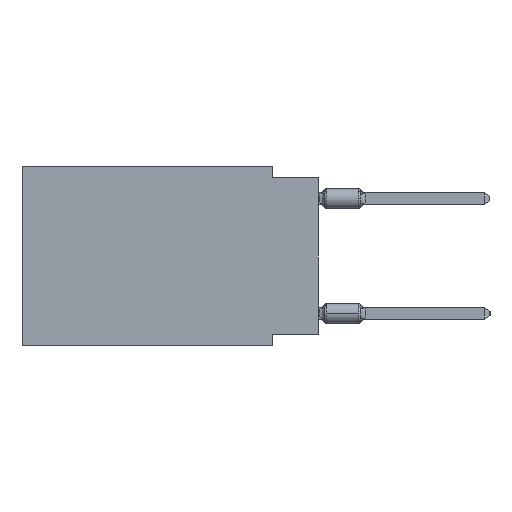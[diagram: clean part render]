
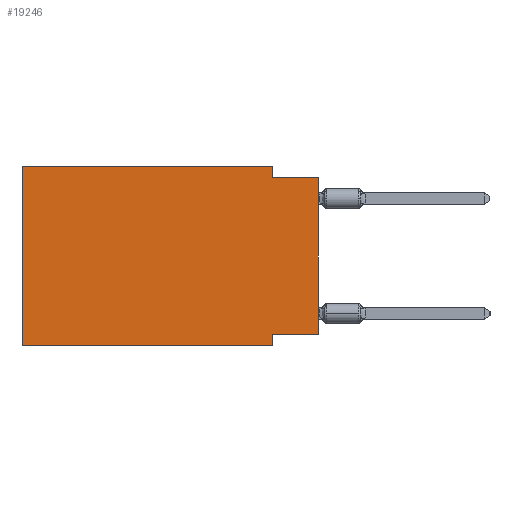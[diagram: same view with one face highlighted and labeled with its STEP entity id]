
A CAD part, left-side view. The second image highlights one B-rep face of the part: STEP entity #19246.
In plain terms, the highlighted planar face has unit normal (-1, 0, 0).
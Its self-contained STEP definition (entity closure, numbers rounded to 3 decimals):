
#781 = DIRECTION ( 'NONE',  ( 0., 1., 0. ) ) ;
#1164 = LINE ( 'NONE', #32238, #18415 ) ;
#2078 = VERTEX_POINT ( 'NONE', #16700 ) ;
#3327 = VERTEX_POINT ( 'NONE', #29608 ) ;
#3727 = CARTESIAN_POINT ( 'NONE',  ( 0., 16.383, -9.906 ) ) ;
#4197 = CARTESIAN_POINT ( 'NONE',  ( 0., 16.383, 0. ) ) ;
#5447 = CARTESIAN_POINT ( 'NONE',  ( 0., 2.54, -9.906 ) ) ;
#6340 = DIRECTION ( 'NONE',  ( 0., -1., 0. ) ) ;
#6601 = EDGE_CURVE ( 'NONE', #8725, #21561, #20114, .T. ) ;
#6744 = CARTESIAN_POINT ( 'NONE',  ( 0., 0., -9.271 ) ) ;
#7801 = CARTESIAN_POINT ( 'NONE',  ( 0., 2.54, 0. ) ) ;
#8725 = VERTEX_POINT ( 'NONE', #10551 ) ;
#9863 = EDGE_CURVE ( 'NONE', #2078, #21561, #28141, .T. ) ;
#9969 = DIRECTION ( 'NONE',  ( 0., 0., 1. ) ) ;
#9999 = EDGE_CURVE ( 'NONE', #13190, #2078, #26656, .T. ) ;
#10115 = VERTEX_POINT ( 'NONE', #18653 ) ;
#10551 = CARTESIAN_POINT ( 'NONE',  ( 0., 16.383, -9.906 ) ) ;
#11182 = VECTOR ( 'NONE', #6340, 1000. ) ;
#12348 = DIRECTION ( 'NONE',  ( 0., 0., 1. ) ) ;
#12403 = PLANE ( 'NONE',  #26948 ) ;
#13190 = VERTEX_POINT ( 'NONE', #34183 ) ;
#13383 = DIRECTION ( 'NONE',  ( 0., 0., -1. ) ) ;
#14023 = CARTESIAN_POINT ( 'NONE',  ( 0., 2.54, -9.906 ) ) ;
#15368 = CARTESIAN_POINT ( 'NONE',  ( 0., 0., -0.635 ) ) ;
#15559 = DIRECTION ( 'NONE',  ( 1., 0., 0. ) ) ;
#15912 = CARTESIAN_POINT ( 'NONE',  ( 0., 0., -0.635 ) ) ;
#16056 = EDGE_CURVE ( 'NONE', #10115, #3327, #20407, .T. ) ;
#16066 = DIRECTION ( 'NONE',  ( 0., -1., 0. ) ) ;
#16265 = DIRECTION ( 'NONE',  ( 0., -1., 0. ) ) ;
#16700 = CARTESIAN_POINT ( 'NONE',  ( 0., 2.54, -9.271 ) ) ;
#16948 = CARTESIAN_POINT ( 'NONE',  ( 0., 2.54, -0.635 ) ) ;
#18415 = VECTOR ( 'NONE', #12348, 1000. ) ;
#18653 = CARTESIAN_POINT ( 'NONE',  ( 0., 16.383, 0. ) ) ;
#19138 = EDGE_CURVE ( 'NONE', #8725, #10115, #35087, .T. ) ;
#19246 = ADVANCED_FACE ( 'NONE', ( #26521 ), #12403, .F. ) ;
#19527 = LINE ( 'NONE', #7801, #29988 ) ;
#20114 = LINE ( 'NONE', #3727, #11182 ) ;
#20407 = LINE ( 'NONE', #29647, #36608 ) ;
#21187 = ORIENTED_EDGE ( 'NONE', *, *, #16056, .F. ) ;
#21561 = VERTEX_POINT ( 'NONE', #5447 ) ;
#22024 = LINE ( 'NONE', #15912, #30311 ) ;
#22177 = VECTOR ( 'NONE', #9969, 1000. ) ;
#22867 = ORIENTED_EDGE ( 'NONE', *, *, #9863, .F. ) ;
#23154 = ORIENTED_EDGE ( 'NONE', *, *, #6601, .T. ) ;
#24070 = VECTOR ( 'NONE', #781, 1000. ) ;
#24175 = ORIENTED_EDGE ( 'NONE', *, *, #9999, .F. ) ;
#25061 = ORIENTED_EDGE ( 'NONE', *, *, #26858, .F. ) ;
#25345 = DIRECTION ( 'NONE',  ( 0., 0., -1. ) ) ;
#26521 = FACE_OUTER_BOUND ( 'NONE', #36058, .T. ) ;
#26656 = LINE ( 'NONE', #6744, #24070 ) ;
#26858 = EDGE_CURVE ( 'NONE', #3327, #35285, #19527, .T. ) ;
#26891 = DIRECTION ( 'NONE',  ( 0., 0., -1. ) ) ;
#26948 = AXIS2_PLACEMENT_3D ( 'NONE', #4197, #15559, #26891 ) ;
#27945 = ORIENTED_EDGE ( 'NONE', *, *, #35835, .F. ) ;
#28141 = LINE ( 'NONE', #14023, #32395 ) ;
#29608 = CARTESIAN_POINT ( 'NONE',  ( 0., 2.54, 0. ) ) ;
#29647 = CARTESIAN_POINT ( 'NONE',  ( 0., 16.383, 0. ) ) ;
#29988 = VECTOR ( 'NONE', #13383, 1000. ) ;
#30311 = VECTOR ( 'NONE', #16265, 1000. ) ;
#32116 = CARTESIAN_POINT ( 'NONE',  ( 0., 16.383, 0. ) ) ;
#32238 = CARTESIAN_POINT ( 'NONE',  ( 0., 0., 0. ) ) ;
#32395 = VECTOR ( 'NONE', #25345, 1000. ) ;
#32682 = ORIENTED_EDGE ( 'NONE', *, *, #34983, .T. ) ;
#34183 = CARTESIAN_POINT ( 'NONE',  ( 0., 0., -9.271 ) ) ;
#34983 = EDGE_CURVE ( 'NONE', #13190, #35748, #1164, .T. ) ;
#35087 = LINE ( 'NONE', #32116, #22177 ) ;
#35285 = VERTEX_POINT ( 'NONE', #16948 ) ;
#35748 = VERTEX_POINT ( 'NONE', #15368 ) ;
#35835 = EDGE_CURVE ( 'NONE', #35285, #35748, #22024, .T. ) ;
#36058 = EDGE_LOOP ( 'NONE', ( #32682, #27945, #25061, #21187, #36799, #23154, #22867, #24175 ) ) ;
#36608 = VECTOR ( 'NONE', #16066, 1000. ) ;
#36799 = ORIENTED_EDGE ( 'NONE', *, *, #19138, .F. ) ;
